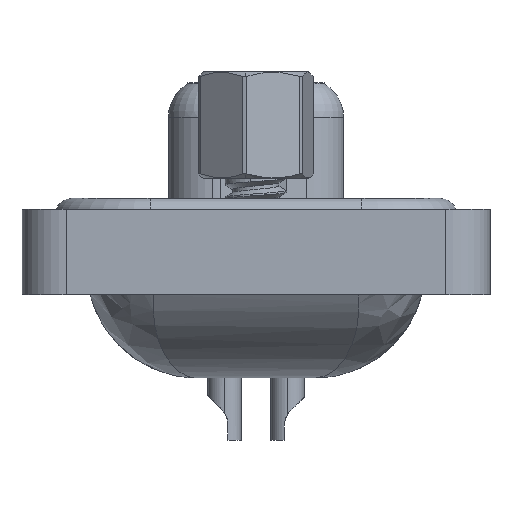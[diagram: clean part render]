
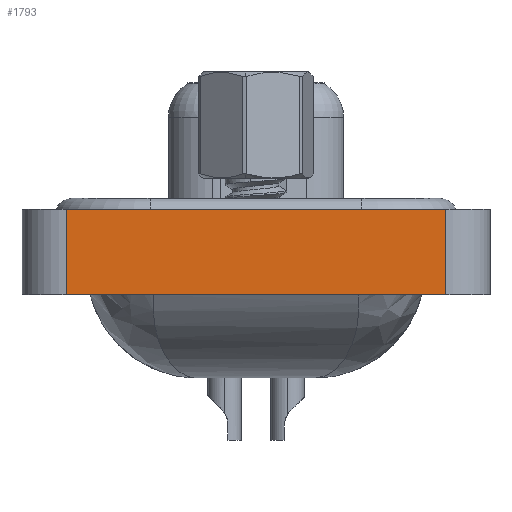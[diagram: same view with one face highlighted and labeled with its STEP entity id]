
A CAD part, left-side view. The second image highlights one B-rep face of the part: STEP entity #1793.
In plain terms, the highlighted planar face has unit normal (-1, 0, 0).
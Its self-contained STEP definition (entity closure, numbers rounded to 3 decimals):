
#156 = EDGE_CURVE ( 'NONE', #869, #5882, #17087, .T. ) ;
#350 = DIRECTION ( 'NONE',  ( 0., -1., 0. ) ) ;
#869 = VERTEX_POINT ( 'NONE', #6484 ) ;
#1793 = ADVANCED_FACE ( 'NONE', ( #8281 ), #18371, .T. ) ;
#1959 = ORIENTED_EDGE ( 'NONE', *, *, #19854, .T. ) ;
#2577 = EDGE_LOOP ( 'NONE', ( #1959, #7329, #3772, #9682 ) ) ;
#3772 = ORIENTED_EDGE ( 'NONE', *, *, #21096, .F. ) ;
#4149 = VERTEX_POINT ( 'NONE', #21742 ) ;
#4752 = DIRECTION ( 'NONE',  ( 0., 0., 1. ) ) ;
#5294 = DIRECTION ( 'NONE',  ( 0., -1., 0. ) ) ;
#5882 = VERTEX_POINT ( 'NONE', #9888 ) ;
#6484 = CARTESIAN_POINT ( 'NONE',  ( -7.25, 8.55, -3.35 ) ) ;
#7329 = ORIENTED_EDGE ( 'NONE', *, *, #14005, .F. ) ;
#7550 = VECTOR ( 'NONE', #350, 1000. ) ;
#8281 = FACE_OUTER_BOUND ( 'NONE', #2577, .T. ) ;
#8537 = CARTESIAN_POINT ( 'NONE',  ( -7.25, 8.55, 0.5 ) ) ;
#8896 = VECTOR ( 'NONE', #5294, 1000. ) ;
#9682 = ORIENTED_EDGE ( 'NONE', *, *, #156, .T. ) ;
#9888 = CARTESIAN_POINT ( 'NONE',  ( -7.25, -8.55, -3.35 ) ) ;
#10046 = CARTESIAN_POINT ( 'NONE',  ( -7.25, -8.55, -3.35 ) ) ;
#10244 = CARTESIAN_POINT ( 'NONE',  ( -7.25, -8.55, 0.5 ) ) ;
#13006 = CARTESIAN_POINT ( 'NONE',  ( -7.25, 8.55, -3.35 ) ) ;
#13566 = CARTESIAN_POINT ( 'NONE',  ( -7.25, -8.55, -3.35 ) ) ;
#14005 = EDGE_CURVE ( 'NONE', #18825, #4149, #20233, .T. ) ;
#14661 = LINE ( 'NONE', #13006, #15910 ) ;
#15081 = DIRECTION ( 'NONE',  ( 0., 0., 1. ) ) ;
#15443 = CARTESIAN_POINT ( 'NONE',  ( -7.25, -8.55, -3.35 ) ) ;
#15910 = VECTOR ( 'NONE', #19678, 1000. ) ;
#16108 = AXIS2_PLACEMENT_3D ( 'NONE', #10046, #16739, #15081 ) ;
#16739 = DIRECTION ( 'NONE',  ( -1., 0., 0. ) ) ;
#16826 = LINE ( 'NONE', #13566, #20812 ) ;
#17087 = LINE ( 'NONE', #15443, #7550 ) ;
#18371 = PLANE ( 'NONE',  #16108 ) ;
#18825 = VERTEX_POINT ( 'NONE', #8537 ) ;
#19678 = DIRECTION ( 'NONE',  ( 0., 0., 1. ) ) ;
#19854 = EDGE_CURVE ( 'NONE', #5882, #4149, #16826, .T. ) ;
#20233 = LINE ( 'NONE', #10244, #8896 ) ;
#20812 = VECTOR ( 'NONE', #4752, 1000. ) ;
#21096 = EDGE_CURVE ( 'NONE', #869, #18825, #14661, .T. ) ;
#21742 = CARTESIAN_POINT ( 'NONE',  ( -7.25, -8.55, 0.5 ) ) ;
